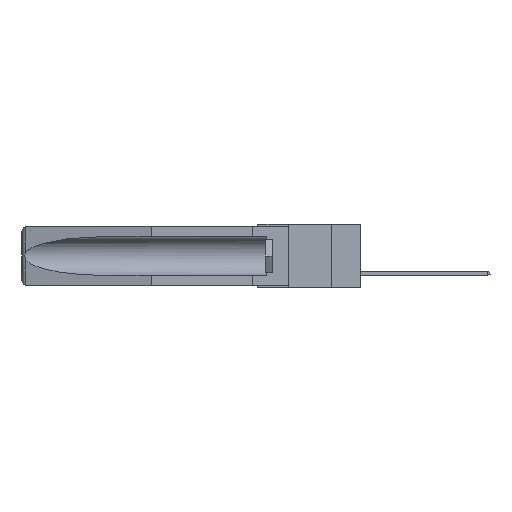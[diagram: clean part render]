
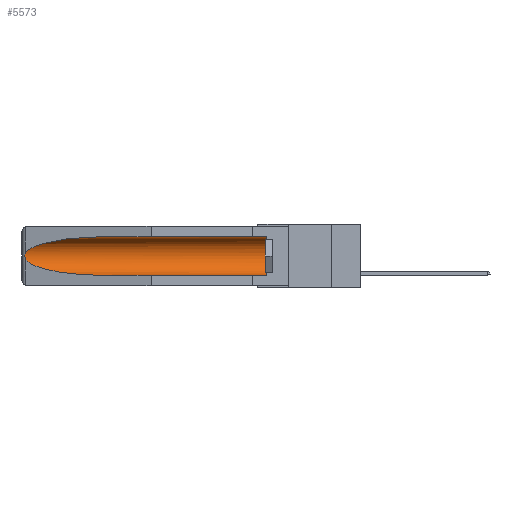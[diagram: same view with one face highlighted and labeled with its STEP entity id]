
A CAD part, left-side view. The second image highlights one B-rep face of the part: STEP entity #5573.
In plain terms, the highlighted cylindrical face has radius 2.857 mm (diameter 5.715 mm), a partial arc.
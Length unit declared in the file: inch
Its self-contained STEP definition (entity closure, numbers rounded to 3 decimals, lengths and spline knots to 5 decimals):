
#55 = CARTESIAN_POINT ( 'NONE',  ( 0.25451, 1.48313, -0.09465 ) ) ;
#485 = EDGE_CURVE ( 'NONE', #8268, #18446, #7306, .T. ) ;
#2251 = B_SPLINE_CURVE_WITH_KNOTS ( 'NONE', 3,
 ( #2472, #15508, #24667, #17550, #17735, #24462, #4474, #4281, #24565, #19977 ),
 .UNSPECIFIED., .F., .F.,
 ( 4, 2, 2, 2, 4 ),
 ( 0., 0.00029, 0.00058, 0.00087, 0.00117 ),
 .UNSPECIFIED. ) ;
#2472 = CARTESIAN_POINT ( 'NONE',  ( 0.26537, 1.52718, -0.14972 ) ) ;
#2861 = DIRECTION ( 'NONE',  ( 0., -1., 0. ) ) ;
#4032 = DIRECTION ( 'NONE',  ( 0., 1., 0. ) ) ;
#4191 = CARTESIAN_POINT ( 'NONE',  ( 0.21114, 1.30732, -0.059 ) ) ;
#4281 = CARTESIAN_POINT ( 'NONE',  ( 0.26655, 1.53094, -0.18657 ) ) ;
#4372 = CARTESIAN_POINT ( 'NONE',  ( 0.155, 1.07973, -0.059 ) ) ;
#4474 = CARTESIAN_POINT ( 'NONE',  ( 0.2673, 1.53269, -0.17917 ) ) ;
#4877 = DIRECTION ( 'NONE',  ( 0., 1., 0. ) ) ;
#5170 = CARTESIAN_POINT ( 'NONE',  ( 0.155, 0.126, -0.1715 ) ) ;
#5573 = ADVANCED_FACE ( 'NONE', ( #18062 ), #13555, .F. ) ;
#5817 = CARTESIAN_POINT ( 'NONE',  ( 0.26537, 1.52718, -0.14972 ) ) ;
#5856 = ORIENTED_EDGE ( 'NONE', *, *, #485, .T. ) ;
#6131 = DIRECTION ( 'NONE',  ( 0., 1., 0. ) ) ;
#6232 = CIRCLE ( 'NONE', #14162, 0.1125 ) ;
#6453 = ORIENTED_EDGE ( 'NONE', *, *, #20475, .T. ) ;
#6634 = CARTESIAN_POINT ( 'NONE',  ( 0.155, 1.07973, -0.284 ) ) ;
#6853 = VERTEX_POINT ( 'NONE', #7554 ) ;
#7306 = LINE ( 'NONE', #28186, #13150 ) ;
#7554 = CARTESIAN_POINT ( 'NONE',  ( 0.155, 1.07973, -0.284 ) ) ;
#8149 = AXIS2_PLACEMENT_3D ( 'NONE', #17644, #4877, #20472 ) ;
#8268 = VERTEX_POINT ( 'NONE', #27419 ) ;
#8586 = EDGE_CURVE ( 'NONE', #18446, #27029, #11656, .T. ) ;
#8829 = EDGE_CURVE ( 'NONE', #23777, #8268, #6232, .T. ) ;
#8874 = EDGE_LOOP ( 'NONE', ( #20830, #6453, #17591, #12747, #17525, #5856 ) ) ;
#9321 = LINE ( 'NONE', #12888, #10326 ) ;
#10326 = VECTOR ( 'NONE', #6131, 39.37008 ) ;
#11634 = VERTEX_POINT ( 'NONE', #18677 ) ;
#11656 =( BOUNDED_CURVE ( )  B_SPLINE_CURVE ( 3, ( #4372, #4191, #55, #17361 ),
 .UNSPECIFIED., .F., .F. ) 
 B_SPLINE_CURVE_WITH_KNOTS ( ( 4, 4 ),
 ( 4.71239, 6.08839 ),
 .UNSPECIFIED. ) 
 CURVE ( )  GEOMETRIC_REPRESENTATION_ITEM ( )  RATIONAL_B_SPLINE_CURVE ( ( 1., 0.848, 0.848, 1. ) ) 
 REPRESENTATION_ITEM ( '' )  );
#11847 = DIRECTION ( 'NONE',  ( 0., 0., 1. ) ) ;
#12539 = EDGE_CURVE ( 'NONE', #23777, #6853, #9321, .T. ) ;
#12747 = ORIENTED_EDGE ( 'NONE', *, *, #12539, .F. ) ;
#12888 = CARTESIAN_POINT ( 'NONE',  ( 0.155, -0.30754, -0.284 ) ) ;
#13150 = VECTOR ( 'NONE', #4032, 39.37008 ) ;
#13555 = CYLINDRICAL_SURFACE ( 'NONE', #8149, 0.1125 ) ;
#13832 = CARTESIAN_POINT ( 'NONE',  ( 0.155, 1.07973, -0.059 ) ) ;
#14162 = AXIS2_PLACEMENT_3D ( 'NONE', #5170, #2861, #11847 ) ;
#15508 = CARTESIAN_POINT ( 'NONE',  ( 0.26597, 1.52961, -0.15275 ) ) ;
#17361 = CARTESIAN_POINT ( 'NONE',  ( 0.26537, 1.52718, -0.14972 ) ) ;
#17525 = ORIENTED_EDGE ( 'NONE', *, *, #8829, .T. ) ;
#17550 = CARTESIAN_POINT ( 'NONE',  ( 0.2673, 1.5327, -0.16383 ) ) ;
#17591 = ORIENTED_EDGE ( 'NONE', *, *, #19018, .T. ) ;
#17644 = CARTESIAN_POINT ( 'NONE',  ( 0.155, -0.30754, -0.1715 ) ) ;
#17735 = CARTESIAN_POINT ( 'NONE',  ( 0.2675, 1.53308, -0.16763 ) ) ;
#18062 = FACE_OUTER_BOUND ( 'NONE', #8874, .T. ) ;
#18446 = VERTEX_POINT ( 'NONE', #13832 ) ;
#18677 = CARTESIAN_POINT ( 'NONE',  ( 0.26537, 1.52718, -0.19328 ) ) ;
#19018 = EDGE_CURVE ( 'NONE', #11634, #6853, #28525, .T. ) ;
#19977 = CARTESIAN_POINT ( 'NONE',  ( 0.26537, 1.52718, -0.19328 ) ) ;
#19988 = CARTESIAN_POINT ( 'NONE',  ( 0.26537, 1.52718, -0.19328 ) ) ;
#20089 = CARTESIAN_POINT ( 'NONE',  ( 0.25451, 1.48313, -0.24835 ) ) ;
#20472 = DIRECTION ( 'NONE',  ( 0., 0., 1. ) ) ;
#20475 = EDGE_CURVE ( 'NONE', #27029, #11634, #2251, .T. ) ;
#20830 = ORIENTED_EDGE ( 'NONE', *, *, #8586, .T. ) ;
#22333 = CARTESIAN_POINT ( 'NONE',  ( 0.21114, 1.30732, -0.284 ) ) ;
#23678 = CARTESIAN_POINT ( 'NONE',  ( 0.155, 0.126, -0.284 ) ) ;
#23777 = VERTEX_POINT ( 'NONE', #23678 ) ;
#24462 = CARTESIAN_POINT ( 'NONE',  ( 0.2675, 1.53308, -0.17534 ) ) ;
#24565 = CARTESIAN_POINT ( 'NONE',  ( 0.26597, 1.5296, -0.19026 ) ) ;
#24667 = CARTESIAN_POINT ( 'NONE',  ( 0.26654, 1.53092, -0.15636 ) ) ;
#27029 = VERTEX_POINT ( 'NONE', #5817 ) ;
#27419 = CARTESIAN_POINT ( 'NONE',  ( 0.155, 0.126, -0.059 ) ) ;
#28186 = CARTESIAN_POINT ( 'NONE',  ( 0.155, -0.30754, -0.059 ) ) ;
#28525 =( BOUNDED_CURVE ( )  B_SPLINE_CURVE ( 3, ( #19988, #20089, #22333, #6634 ),
 .UNSPECIFIED., .F., .F. ) 
 B_SPLINE_CURVE_WITH_KNOTS ( ( 4, 4 ),
 ( 0.1948, 1.5708 ),
 .UNSPECIFIED. ) 
 CURVE ( )  GEOMETRIC_REPRESENTATION_ITEM ( )  RATIONAL_B_SPLINE_CURVE ( ( 1., 0.848, 0.848, 1. ) ) 
 REPRESENTATION_ITEM ( '' )  );
